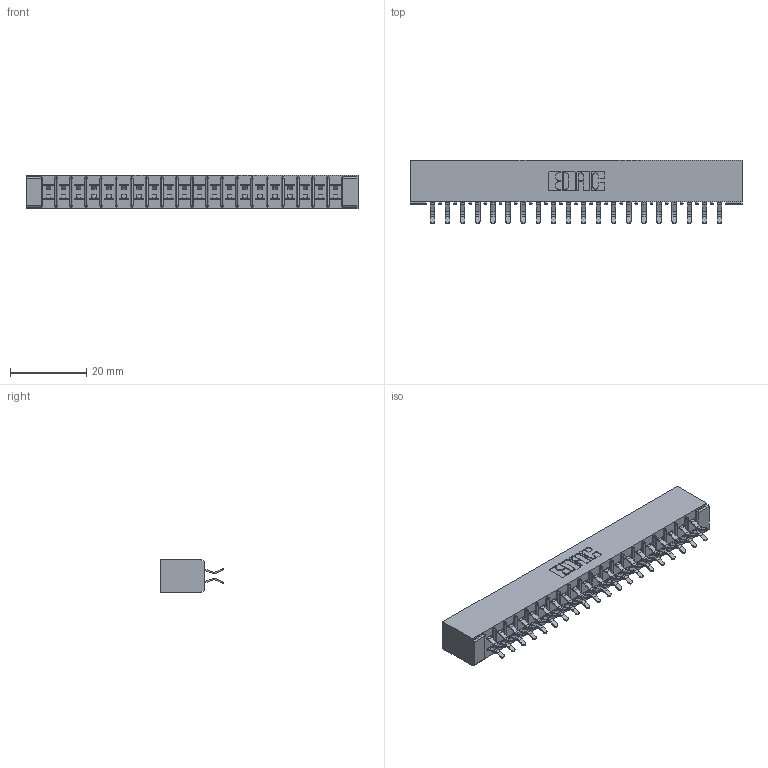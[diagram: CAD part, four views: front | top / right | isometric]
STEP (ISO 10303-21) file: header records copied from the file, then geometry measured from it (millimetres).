
FILE_DESCRIPTION (( 'STEP AP203' ), '1' );
FILE_NAME ('315-040-556-201.STEP', '2019-09-10T17:24:16', ( '' ), ( '' ), 'SwSTEP 2.0', 'SolidWorks 2016', '' );
FILE_SCHEMA (( 'CONFIG_CONTROL_DESIGN' ));
Length unit declared in the file: inch
Products named in the file (3): 305 Part_No Mounting; 315-040-556-201; 305-290-001_556
Assembly tree (41 placements, depth 2):
  315-040-556-201
    305 Part_No Mounting
    305-290-001_556  x40
Bounding box: 87.12 x 16.64 x 8.71 mm (x, y, z)
Volume: 5655.7 mm3; surface area: 11130.9 mm2
Topology: 41 solids, 41 shells, 2348 faces, 6752 edges, 4392 vertices
Faces by surface type: plane 1304, cylinder 964, sphere 80
Entity records: 24277 total; most frequent: CARTESIAN_POINT 4018, ORIENTED_EDGE 3984, DIRECTION 3906, EDGE_CURVE 1992, LINE 1586, VECTOR 1586, VERTEX_POINT 1272, AXIS2_PLACEMENT_3D 1160
